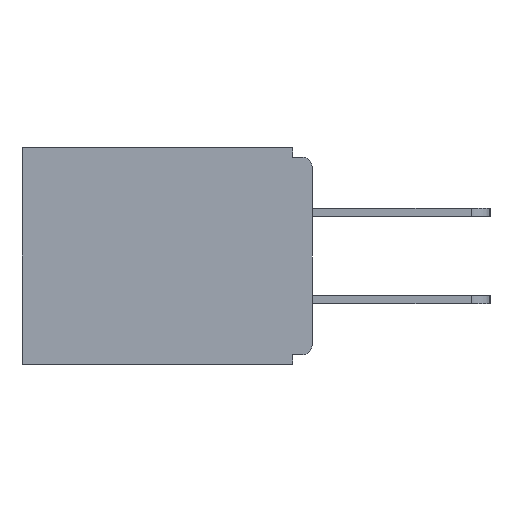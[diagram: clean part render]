
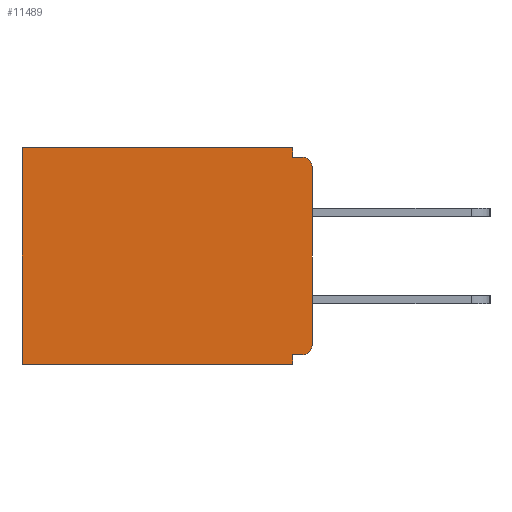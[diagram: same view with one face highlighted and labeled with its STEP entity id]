
A CAD part, left-side view. The second image highlights one B-rep face of the part: STEP entity #11489.
In plain terms, the highlighted planar face has unit normal (-1, 0, 0).
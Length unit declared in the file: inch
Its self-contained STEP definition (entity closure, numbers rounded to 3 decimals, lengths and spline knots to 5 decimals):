
#13 = LINE ( 'NONE', #13283, #7973 ) ;
#260 = VECTOR ( 'NONE', #13515, 39.37008 ) ;
#370 = CARTESIAN_POINT ( 'NONE',  ( 0.298, 0.031, -0.015 ) ) ;
#397 = CIRCLE ( 'NONE', #10099, 0.015 ) ;
#441 = VERTEX_POINT ( 'NONE', #10497 ) ;
#801 = LINE ( 'NONE', #7610, #11506 ) ;
#868 = VECTOR ( 'NONE', #3280, 39.37008 ) ;
#1089 = DIRECTION ( 'NONE',  ( 0., -1., 0. ) ) ;
#1554 = VERTEX_POINT ( 'NONE', #11967 ) ;
#1985 = EDGE_CURVE ( 'NONE', #10980, #16211, #7383, .T. ) ;
#2396 = CARTESIAN_POINT ( 'NONE',  ( 0.298, 0.031, -0.343 ) ) ;
#2707 = CARTESIAN_POINT ( 'NONE',  ( 0.298, 0., -0.328 ) ) ;
#2749 = DIRECTION ( 'NONE',  ( 0., 0., -1. ) ) ;
#2836 = EDGE_CURVE ( 'NONE', #16211, #6060, #13, .T. ) ;
#3150 = EDGE_CURVE ( 'NONE', #16421, #1554, #801, .T. ) ;
#3186 = DIRECTION ( 'NONE',  ( 0., 0., -1. ) ) ;
#3280 = DIRECTION ( 'NONE',  ( 0., 0., -1. ) ) ;
#3380 = CIRCLE ( 'NONE', #15500, 0.015 ) ;
#3488 = EDGE_CURVE ( 'NONE', #6107, #9944, #13822, .T. ) ;
#3841 = ORIENTED_EDGE ( 'NONE', *, *, #2836, .T. ) ;
#3891 = DIRECTION ( 'NONE',  ( -1., 0., 0. ) ) ;
#4004 = AXIS2_PLACEMENT_3D ( 'NONE', #13092, #4866, #15749 ) ;
#4239 = CARTESIAN_POINT ( 'NONE',  ( 0.298, 0.031, -0.343 ) ) ;
#4466 = CARTESIAN_POINT ( 'NONE',  ( 0.298, 0., -0.343 ) ) ;
#4630 = EDGE_CURVE ( 'NONE', #9944, #5869, #5153, .T. ) ;
#4866 = DIRECTION ( 'NONE',  ( 1., 0., 0. ) ) ;
#5153 = LINE ( 'NONE', #2396, #11883 ) ;
#5161 = ORIENTED_EDGE ( 'NONE', *, *, #6868, .F. ) ;
#5390 = CARTESIAN_POINT ( 'NONE',  ( 0.298, 0., -0.313 ) ) ;
#5398 = LINE ( 'NONE', #4466, #6461 ) ;
#5603 = CARTESIAN_POINT ( 'NONE',  ( 0.298, 0.015, -0.328 ) ) ;
#5716 = ORIENTED_EDGE ( 'NONE', *, *, #1985, .T. ) ;
#5869 = VERTEX_POINT ( 'NONE', #16655 ) ;
#6060 = VERTEX_POINT ( 'NONE', #8308 ) ;
#6107 = VERTEX_POINT ( 'NONE', #5603 ) ;
#6159 = ORIENTED_EDGE ( 'NONE', *, *, #3488, .F. ) ;
#6170 = DIRECTION ( 'NONE',  ( 0., 1., 0. ) ) ;
#6461 = VECTOR ( 'NONE', #6170, 39.37008 ) ;
#6512 = CARTESIAN_POINT ( 'NONE',  ( 0.298, 0.031, 0. ) ) ;
#6765 = EDGE_CURVE ( 'NONE', #6107, #16304, #397, .T. ) ;
#6868 = EDGE_CURVE ( 'NONE', #5869, #6060, #5398, .T. ) ;
#7206 = ORIENTED_EDGE ( 'NONE', *, *, #6765, .T. ) ;
#7383 = LINE ( 'NONE', #14751, #260 ) ;
#7596 = LINE ( 'NONE', #12788, #868 ) ;
#7610 = CARTESIAN_POINT ( 'NONE',  ( 0.298, 0., -0.015 ) ) ;
#7823 = DIRECTION ( 'NONE',  ( 0., 0., -1. ) ) ;
#7973 = VECTOR ( 'NONE', #7823, 39.37008 ) ;
#8190 = ORIENTED_EDGE ( 'NONE', *, *, #12683, .T. ) ;
#8266 = DIRECTION ( 'NONE',  ( -1., 0., 0. ) ) ;
#8308 = CARTESIAN_POINT ( 'NONE',  ( 0.298, 0.46, -0.343 ) ) ;
#8705 = EDGE_CURVE ( 'NONE', #10980, #16421, #10818, .T. ) ;
#9609 = ORIENTED_EDGE ( 'NONE', *, *, #3150, .F. ) ;
#9944 = VERTEX_POINT ( 'NONE', #12285 ) ;
#10099 = AXIS2_PLACEMENT_3D ( 'NONE', #13171, #3891, #3186 ) ;
#10433 = ORIENTED_EDGE ( 'NONE', *, *, #4630, .F. ) ;
#10497 = CARTESIAN_POINT ( 'NONE',  ( 0.298, 0., -0.03 ) ) ;
#10563 = CARTESIAN_POINT ( 'NONE',  ( 0.298, 0.46, 0. ) ) ;
#10575 = EDGE_CURVE ( 'NONE', #441, #16304, #7596, .T. ) ;
#10608 = DIRECTION ( 'NONE',  ( 0., 0., -1. ) ) ;
#10818 = LINE ( 'NONE', #4239, #12494 ) ;
#10878 = DIRECTION ( 'NONE',  ( 0., 0., -1. ) ) ;
#10980 = VERTEX_POINT ( 'NONE', #6512 ) ;
#11489 = ADVANCED_FACE ( 'NONE', ( #17069 ), #16906, .F. ) ;
#11506 = VECTOR ( 'NONE', #1089, 39.37008 ) ;
#11883 = VECTOR ( 'NONE', #10608, 39.37008 ) ;
#11967 = CARTESIAN_POINT ( 'NONE',  ( 0.298, 0.015, -0.015 ) ) ;
#12093 = DIRECTION ( 'NONE',  ( 0., 1., 0. ) ) ;
#12285 = CARTESIAN_POINT ( 'NONE',  ( 0.298, 0.031, -0.328 ) ) ;
#12494 = VECTOR ( 'NONE', #10878, 39.37008 ) ;
#12683 = EDGE_CURVE ( 'NONE', #441, #1554, #3380, .T. ) ;
#12784 = ORIENTED_EDGE ( 'NONE', *, *, #8705, .F. ) ;
#12788 = CARTESIAN_POINT ( 'NONE',  ( 0.298, 0., 0. ) ) ;
#13092 = CARTESIAN_POINT ( 'NONE',  ( 0.298, 0., 0. ) ) ;
#13171 = CARTESIAN_POINT ( 'NONE',  ( 0.298, 0.015, -0.313 ) ) ;
#13283 = CARTESIAN_POINT ( 'NONE',  ( 0.298, 0.46, 0. ) ) ;
#13381 = CARTESIAN_POINT ( 'NONE',  ( 0.298, 0.015, -0.03 ) ) ;
#13515 = DIRECTION ( 'NONE',  ( 0., 1., 0. ) ) ;
#13769 = EDGE_LOOP ( 'NONE', ( #8190, #9609, #12784, #5716, #3841, #5161, #10433, #6159, #7206, #16647 ) ) ;
#13822 = LINE ( 'NONE', #2707, #14023 ) ;
#14023 = VECTOR ( 'NONE', #12093, 39.37008 ) ;
#14751 = CARTESIAN_POINT ( 'NONE',  ( 0.298, 0., 0. ) ) ;
#15500 = AXIS2_PLACEMENT_3D ( 'NONE', #13381, #8266, #2749 ) ;
#15749 = DIRECTION ( 'NONE',  ( 0., 0., -1. ) ) ;
#16211 = VERTEX_POINT ( 'NONE', #10563 ) ;
#16304 = VERTEX_POINT ( 'NONE', #5390 ) ;
#16421 = VERTEX_POINT ( 'NONE', #370 ) ;
#16647 = ORIENTED_EDGE ( 'NONE', *, *, #10575, .F. ) ;
#16655 = CARTESIAN_POINT ( 'NONE',  ( 0.298, 0.031, -0.343 ) ) ;
#16906 = PLANE ( 'NONE',  #4004 ) ;
#17069 = FACE_OUTER_BOUND ( 'NONE', #13769, .T. ) ;
